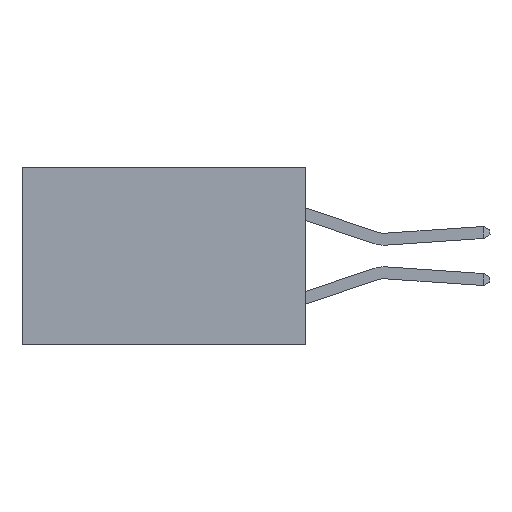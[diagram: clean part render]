
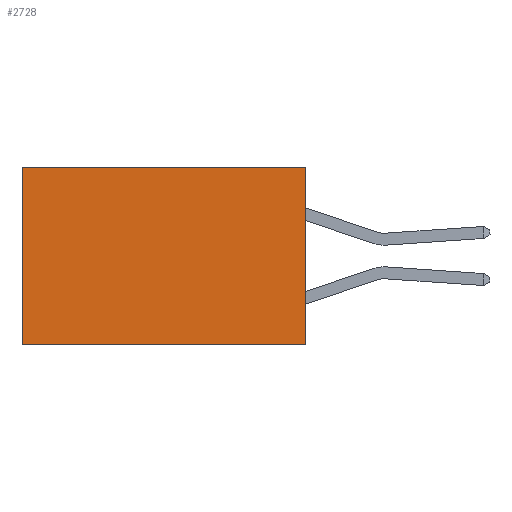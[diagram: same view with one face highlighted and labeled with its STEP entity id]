
A CAD part, left-side view. The second image highlights one B-rep face of the part: STEP entity #2728.
In plain terms, the highlighted planar face has unit normal (-1, 0, 0).
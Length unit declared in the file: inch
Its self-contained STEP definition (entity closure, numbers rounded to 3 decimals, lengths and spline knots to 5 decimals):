
#37 = EDGE_CURVE ( 'NONE', #3136, #4950, #4572, .T. ) ;
#160 = VECTOR ( 'NONE', #6792, 39.37008 ) ;
#231 = EDGE_CURVE ( 'NONE', #4950, #3451, #2300, .T. ) ;
#304 = DIRECTION ( 'NONE',  ( 1., 0., 0. ) ) ;
#569 = VECTOR ( 'NONE', #7420, 39.37008 ) ;
#1451 = CARTESIAN_POINT ( 'NONE',  ( 0.277, 0., -0.37 ) ) ;
#1534 = ORIENTED_EDGE ( 'NONE', *, *, #3693, .F. ) ;
#1790 = DIRECTION ( 'NONE',  ( 0., 1., 0. ) ) ;
#1946 = LINE ( 'NONE', #6882, #160 ) ;
#2300 = LINE ( 'NONE', #8331, #5680 ) ;
#2456 = DIRECTION ( 'NONE',  ( 0., 0., -1. ) ) ;
#2538 = LINE ( 'NONE', #7721, #569 ) ;
#2553 = FACE_OUTER_BOUND ( 'NONE', #4349, .T. ) ;
#2728 = ADVANCED_FACE ( 'NONE', ( #2553 ), #6925, .F. ) ;
#3136 = VERTEX_POINT ( 'NONE', #6102 ) ;
#3229 = ORIENTED_EDGE ( 'NONE', *, *, #37, .T. ) ;
#3451 = VERTEX_POINT ( 'NONE', #6920 ) ;
#3638 = EDGE_CURVE ( 'NONE', #3782, #3451, #2538, .T. ) ;
#3693 = EDGE_CURVE ( 'NONE', #3136, #3782, #1946, .T. ) ;
#3782 = VERTEX_POINT ( 'NONE', #5922 ) ;
#4349 = EDGE_LOOP ( 'NONE', ( #4812, #6700, #1534, #3229 ) ) ;
#4368 = VECTOR ( 'NONE', #1790, 39.37008 ) ;
#4390 = CARTESIAN_POINT ( 'NONE',  ( 0.277, 0.59, 0. ) ) ;
#4572 = LINE ( 'NONE', #8301, #4368 ) ;
#4731 = DIRECTION ( 'NONE',  ( 0., 0., -1. ) ) ;
#4812 = ORIENTED_EDGE ( 'NONE', *, *, #231, .T. ) ;
#4950 = VERTEX_POINT ( 'NONE', #4390 ) ;
#5680 = VECTOR ( 'NONE', #4731, 39.37008 ) ;
#5922 = CARTESIAN_POINT ( 'NONE',  ( 0.277, 0., -0.37 ) ) ;
#6102 = CARTESIAN_POINT ( 'NONE',  ( 0.277, 0., 0. ) ) ;
#6700 = ORIENTED_EDGE ( 'NONE', *, *, #3638, .F. ) ;
#6792 = DIRECTION ( 'NONE',  ( 0., 0., -1. ) ) ;
#6882 = CARTESIAN_POINT ( 'NONE',  ( 0.277, 0., -0.37 ) ) ;
#6920 = CARTESIAN_POINT ( 'NONE',  ( 0.277, 0.59, -0.37 ) ) ;
#6925 = PLANE ( 'NONE',  #8371 ) ;
#7420 = DIRECTION ( 'NONE',  ( 0., 1., 0. ) ) ;
#7721 = CARTESIAN_POINT ( 'NONE',  ( 0.277, 0., -0.37 ) ) ;
#8301 = CARTESIAN_POINT ( 'NONE',  ( 0.277, 0., 0. ) ) ;
#8331 = CARTESIAN_POINT ( 'NONE',  ( 0.277, 0.59, -0.37 ) ) ;
#8371 = AXIS2_PLACEMENT_3D ( 'NONE', #1451, #304, #2456 ) ;
